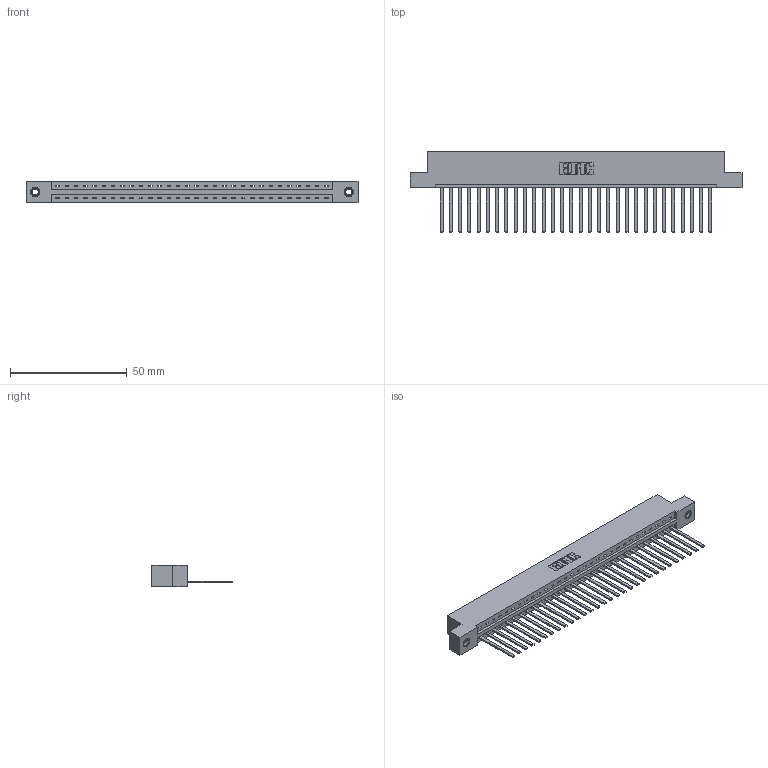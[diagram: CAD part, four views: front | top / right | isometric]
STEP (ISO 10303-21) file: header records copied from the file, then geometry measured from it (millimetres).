
FILE_DESCRIPTION (( 'STEP AP203' ), '1' );
FILE_NAME ('387-030-544-107.STEP', '2019-10-03T18:33:10', ( '' ), ( '' ), 'SwSTEP 2.0', 'SolidWorks 2016', '' );
FILE_SCHEMA (( 'CONFIG_CONTROL_DESIGN' ));
Length unit declared in the file: inch
Products named in the file (4): 387-030-544-107; 345-250-001_345-250-005-103; 345-292-001_345-293-144; 337 Part_Flush Mounting Lugs - 0.156 Dia-TI
Assembly tree (33 placements, depth 2):
  387-030-544-107
    337 Part_Flush Mounting Lugs - 0.156 Dia-TI
    345-292-001_345-293-144  x30
    345-250-001_345-250-005-103  x2
Bounding box: 141.88 x 34.3 x 9.4 mm (x, y, z)
Volume: 14930.3 mm3; surface area: 16545.6 mm2
Topology: 33 solids, 33 shells, 1854 faces, 5547 edges, 3650 vertices
Faces by surface type: plane 1362, cylinder 476, cone 12, torus 4
Entity records: 24854 total; most frequent: CARTESIAN_POINT 4307, ORIENTED_EDGE 4266, DIRECTION 3679, EDGE_CURVE 2133, VECTOR 1989, LINE 1989, VERTEX_POINT 1416, AXIS2_PLACEMENT_3D 845
